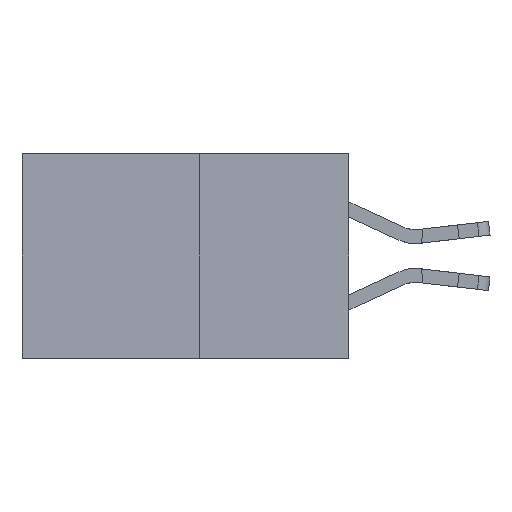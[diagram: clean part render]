
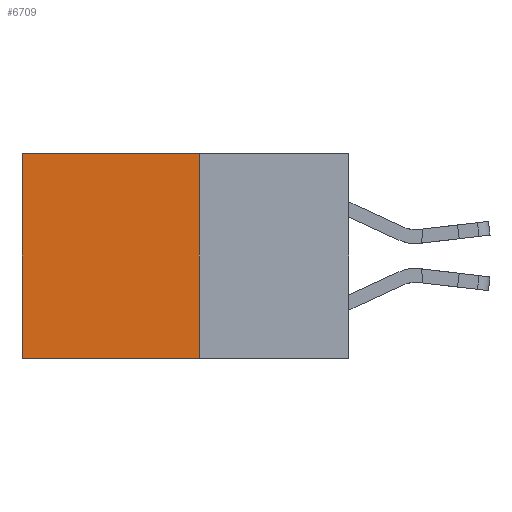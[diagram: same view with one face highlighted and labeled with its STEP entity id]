
A CAD part, left-side view. The second image highlights one B-rep face of the part: STEP entity #6709.
In plain terms, the highlighted planar face has unit normal (-1, 0, 0).
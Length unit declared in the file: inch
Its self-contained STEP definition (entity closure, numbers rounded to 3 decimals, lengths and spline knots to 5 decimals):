
#159 = VERTEX_POINT ( 'NONE', #11402 ) ;
#1724 = EDGE_CURVE ( 'NONE', #2482, #10667, #1991, .T. ) ;
#1991 = LINE ( 'NONE', #14758, #12857 ) ;
#2482 = VERTEX_POINT ( 'NONE', #16905 ) ;
#3013 = EDGE_CURVE ( 'NONE', #159, #10667, #14360, .T. ) ;
#3303 = LINE ( 'NONE', #8253, #10866 ) ;
#3673 = VERTEX_POINT ( 'NONE', #8513 ) ;
#3708 = DIRECTION ( 'NONE',  ( 1., 0., 0. ) ) ;
#5880 = VECTOR ( 'NONE', #15230, 39.37008 ) ;
#6549 = ORIENTED_EDGE ( 'NONE', *, *, #1724, .F. ) ;
#6709 = ADVANCED_FACE ( 'NONE', ( #15559 ), #14926, .F. ) ;
#7537 = ORIENTED_EDGE ( 'NONE', *, *, #11390, .T. ) ;
#7939 = CARTESIAN_POINT ( 'NONE',  ( 0.277, 0.27, -0.37 ) ) ;
#8222 = EDGE_CURVE ( 'NONE', #3673, #2482, #9668, .T. ) ;
#8253 = CARTESIAN_POINT ( 'NONE',  ( 0.277, 0.27, 0. ) ) ;
#8513 = CARTESIAN_POINT ( 'NONE',  ( 0.277, 0.27, 0. ) ) ;
#9668 = LINE ( 'NONE', #13860, #5880 ) ;
#10651 = VECTOR ( 'NONE', #17121, 39.37008 ) ;
#10667 = VERTEX_POINT ( 'NONE', #15172 ) ;
#10866 = VECTOR ( 'NONE', #16576, 39.37008 ) ;
#11390 = EDGE_CURVE ( 'NONE', #3673, #159, #3303, .T. ) ;
#11402 = CARTESIAN_POINT ( 'NONE',  ( 0.277, 0.59, 0. ) ) ;
#12329 = ORIENTED_EDGE ( 'NONE', *, *, #3013, .T. ) ;
#12857 = VECTOR ( 'NONE', #15624, 39.37008 ) ;
#13614 = DIRECTION ( 'NONE',  ( 0., 0., -1. ) ) ;
#13860 = CARTESIAN_POINT ( 'NONE',  ( 0.277, 0.27, -0.37 ) ) ;
#14170 = EDGE_LOOP ( 'NONE', ( #12329, #6549, #16862, #7537 ) ) ;
#14360 = LINE ( 'NONE', #17218, #10651 ) ;
#14758 = CARTESIAN_POINT ( 'NONE',  ( 0.277, 0.27, -0.37 ) ) ;
#14926 = PLANE ( 'NONE',  #16591 ) ;
#15172 = CARTESIAN_POINT ( 'NONE',  ( 0.277, 0.59, -0.37 ) ) ;
#15230 = DIRECTION ( 'NONE',  ( 0., 0., -1. ) ) ;
#15559 = FACE_OUTER_BOUND ( 'NONE', #14170, .T. ) ;
#15624 = DIRECTION ( 'NONE',  ( 0., 1., 0. ) ) ;
#16576 = DIRECTION ( 'NONE',  ( 0., 1., 0. ) ) ;
#16591 = AXIS2_PLACEMENT_3D ( 'NONE', #7939, #3708, #13614 ) ;
#16862 = ORIENTED_EDGE ( 'NONE', *, *, #8222, .F. ) ;
#16905 = CARTESIAN_POINT ( 'NONE',  ( 0.277, 0.27, -0.37 ) ) ;
#17121 = DIRECTION ( 'NONE',  ( 0., 0., -1. ) ) ;
#17218 = CARTESIAN_POINT ( 'NONE',  ( 0.277, 0.59, -0.37 ) ) ;
